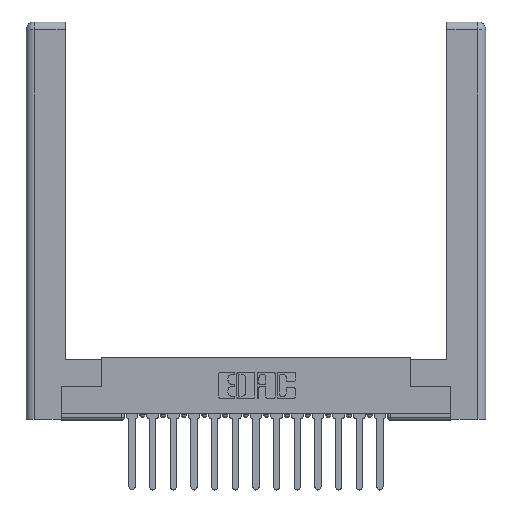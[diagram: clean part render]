
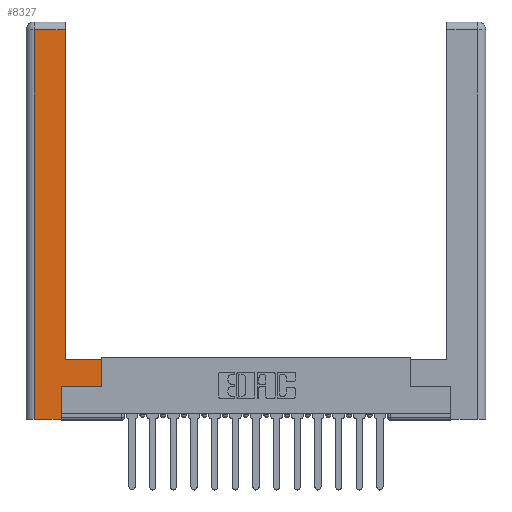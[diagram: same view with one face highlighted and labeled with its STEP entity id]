
A CAD part, top view. The second image highlights one B-rep face of the part: STEP entity #8327.
In plain terms, the highlighted planar face has unit normal (0, 0, 1).
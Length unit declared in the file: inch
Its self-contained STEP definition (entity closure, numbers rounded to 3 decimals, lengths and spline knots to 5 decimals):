
#507 = EDGE_CURVE ( 'NONE', #15742, #8647, #7823, .T. ) ;
#758 = CARTESIAN_POINT ( 'NONE',  ( 0., 0., 0. ) ) ;
#1300 = VERTEX_POINT ( 'NONE', #14617 ) ;
#1439 = VECTOR ( 'NONE', #1644, 39.37008 ) ;
#1623 = DIRECTION ( 'NONE',  ( 0., 1., 0. ) ) ;
#1644 = DIRECTION ( 'NONE',  ( 0., -1., 0. ) ) ;
#1727 = CARTESIAN_POINT ( 'NONE',  ( 0.295, 0.45, 0. ) ) ;
#2054 = ORIENTED_EDGE ( 'NONE', *, *, #7055, .T. ) ;
#2055 = VECTOR ( 'NONE', #7248, 39.37008 ) ;
#2188 = CARTESIAN_POINT ( 'NONE',  ( 0.265, 0., 0. ) ) ;
#2351 = DIRECTION ( 'NONE',  ( 0., 1., 0. ) ) ;
#2414 = EDGE_LOOP ( 'NONE', ( #2054, #14575, #16181, #10261, #11397, #3422, #6481, #9673 ) ) ;
#2859 = DIRECTION ( 'NONE',  ( -1., 0., 0. ) ) ;
#3422 = ORIENTED_EDGE ( 'NONE', *, *, #10397, .T. ) ;
#3463 = EDGE_CURVE ( 'NONE', #8647, #17087, #10195, .T. ) ;
#3896 = DIRECTION ( 'NONE',  ( 1., 0., 0. ) ) ;
#4387 = VERTEX_POINT ( 'NONE', #16728 ) ;
#5223 = VECTOR ( 'NONE', #5910, 39.37008 ) ;
#5910 = DIRECTION ( 'NONE',  ( 1., 0., 0. ) ) ;
#6481 = ORIENTED_EDGE ( 'NONE', *, *, #15620, .T. ) ;
#6668 = CARTESIAN_POINT ( 'NONE',  ( 0.0615, 0., 0. ) ) ;
#7055 = EDGE_CURVE ( 'NONE', #1300, #14404, #10390, .T. ) ;
#7248 = DIRECTION ( 'NONE',  ( -1., 0., 0. ) ) ;
#7374 = VECTOR ( 'NONE', #2351, 39.37008 ) ;
#7427 = EDGE_CURVE ( 'NONE', #4387, #1300, #16627, .T. ) ;
#7484 = PLANE ( 'NONE',  #14338 ) ;
#7556 = VECTOR ( 'NONE', #8249, 39.37008 ) ;
#7823 = LINE ( 'NONE', #15480, #1439 ) ;
#8249 = DIRECTION ( 'NONE',  ( 0., 1., 0. ) ) ;
#8327 = ADVANCED_FACE ( 'NONE', ( #11986 ), #7484, .F. ) ;
#8376 = CARTESIAN_POINT ( 'NONE',  ( 0.0615, 2.94, 0. ) ) ;
#8413 = CARTESIAN_POINT ( 'NONE',  ( 0.565, 0.45, 0. ) ) ;
#8647 = VERTEX_POINT ( 'NONE', #6668 ) ;
#8702 = CARTESIAN_POINT ( 'NONE',  ( 0.295, 2.94, 0. ) ) ;
#8832 = CARTESIAN_POINT ( 'NONE',  ( 0.0615, 2.94, 0. ) ) ;
#9109 = VECTOR ( 'NONE', #2859, 39.37008 ) ;
#9200 = CARTESIAN_POINT ( 'NONE',  ( 0.295, 3., 0. ) ) ;
#9251 = CARTESIAN_POINT ( 'NONE',  ( 0.265, 0., 0. ) ) ;
#9315 = EDGE_CURVE ( 'NONE', #14404, #15742, #13393, .T. ) ;
#9601 = EDGE_CURVE ( 'NONE', #17087, #11661, #10364, .T. ) ;
#9673 = ORIENTED_EDGE ( 'NONE', *, *, #7427, .T. ) ;
#10195 = LINE ( 'NONE', #9251, #13231 ) ;
#10261 = ORIENTED_EDGE ( 'NONE', *, *, #3463, .T. ) ;
#10364 = LINE ( 'NONE', #12373, #7556 ) ;
#10390 = LINE ( 'NONE', #9200, #7374 ) ;
#10397 = EDGE_CURVE ( 'NONE', #11661, #17708, #16167, .T. ) ;
#11397 = ORIENTED_EDGE ( 'NONE', *, *, #9601, .T. ) ;
#11534 = CARTESIAN_POINT ( 'NONE',  ( 0.565, 0.245, 0. ) ) ;
#11661 = VERTEX_POINT ( 'NONE', #12356 ) ;
#11986 = FACE_OUTER_BOUND ( 'NONE', #2414, .T. ) ;
#12356 = CARTESIAN_POINT ( 'NONE',  ( 0.265, 0.245, 0. ) ) ;
#12373 = CARTESIAN_POINT ( 'NONE',  ( 0.265, 0.245, 0. ) ) ;
#12538 = VECTOR ( 'NONE', #1623, 39.37008 ) ;
#13231 = VECTOR ( 'NONE', #3896, 39.37008 ) ;
#13393 = LINE ( 'NONE', #8376, #9109 ) ;
#13818 = LINE ( 'NONE', #8413, #12538 ) ;
#14261 = CARTESIAN_POINT ( 'NONE',  ( 0.565, 0.245, 0. ) ) ;
#14338 = AXIS2_PLACEMENT_3D ( 'NONE', #758, #17131, #15697 ) ;
#14404 = VERTEX_POINT ( 'NONE', #8702 ) ;
#14575 = ORIENTED_EDGE ( 'NONE', *, *, #9315, .T. ) ;
#14617 = CARTESIAN_POINT ( 'NONE',  ( 0.295, 0.45, 0. ) ) ;
#15480 = CARTESIAN_POINT ( 'NONE',  ( 0.0615, 0., 0. ) ) ;
#15620 = EDGE_CURVE ( 'NONE', #17708, #4387, #13818, .T. ) ;
#15697 = DIRECTION ( 'NONE',  ( -1., 0., 0. ) ) ;
#15742 = VERTEX_POINT ( 'NONE', #8832 ) ;
#16167 = LINE ( 'NONE', #14261, #5223 ) ;
#16181 = ORIENTED_EDGE ( 'NONE', *, *, #507, .T. ) ;
#16627 = LINE ( 'NONE', #1727, #2055 ) ;
#16728 = CARTESIAN_POINT ( 'NONE',  ( 0.565, 0.45, 0. ) ) ;
#17087 = VERTEX_POINT ( 'NONE', #2188 ) ;
#17131 = DIRECTION ( 'NONE',  ( 0., 0., -1. ) ) ;
#17708 = VERTEX_POINT ( 'NONE', #11534 ) ;
